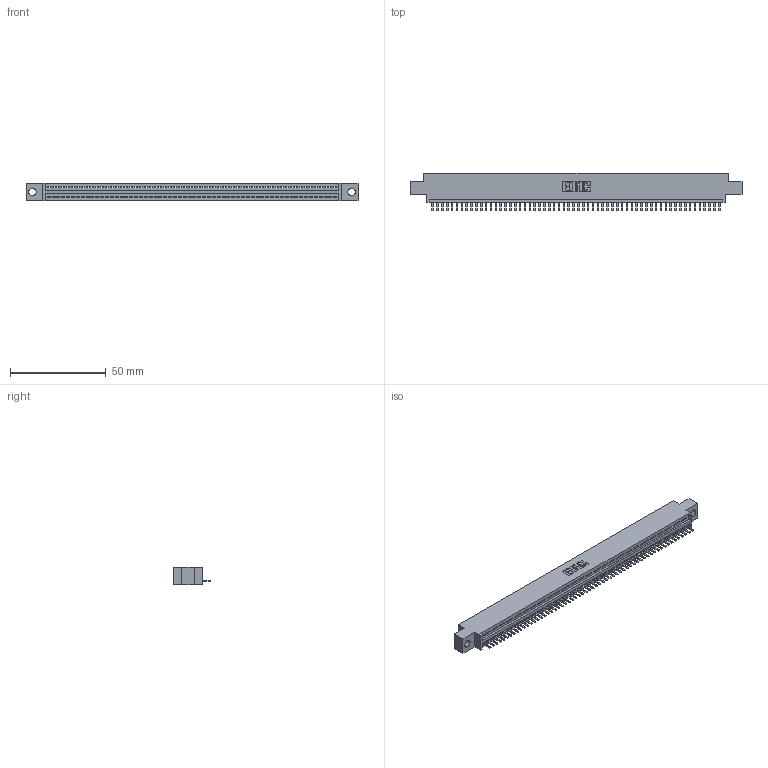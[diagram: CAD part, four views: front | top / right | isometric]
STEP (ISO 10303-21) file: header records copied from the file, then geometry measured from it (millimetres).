
FILE_DESCRIPTION (( 'STEP AP203' ), '1' );
FILE_NAME ('345-060-520-604.STEP', '2021-05-28T15:47:41', ( '' ), ( '' ), 'SwSTEP 2.0', 'SolidWorks 2020', '' );
FILE_SCHEMA (( 'CONFIG_CONTROL_DESIGN' ));
Length unit declared in the file: inch
Products named in the file (3): 345-060-520-604; 345 Part_0.170 Offset - 0.156 Dia-TI; 345-292-001_345-293-120
Assembly tree (61 placements, depth 2):
  345-060-520-604
    345 Part_0.170 Offset - 0.156 Dia-TI
    345-292-001_345-293-120  x60
Bounding box: 173.61 x 19.68 x 9.4 mm (x, y, z)
Volume: 16245.1 mm3; surface area: 21237.3 mm2
Topology: 61 solids, 61 shells, 3864 faces, 11429 edges, 7458 vertices
Faces by surface type: plane 2618, cylinder 1246
Entity records: 43399 total; most frequent: CARTESIAN_POINT 7538, ORIENTED_EDGE 7518, DIRECTION 6543, EDGE_CURVE 3759, VECTOR 3383, LINE 3383, VERTEX_POINT 2502, AXIS2_PLACEMENT_3D 1580
